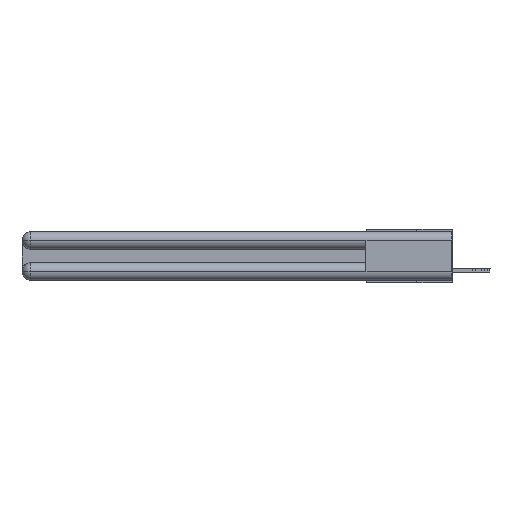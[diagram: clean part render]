
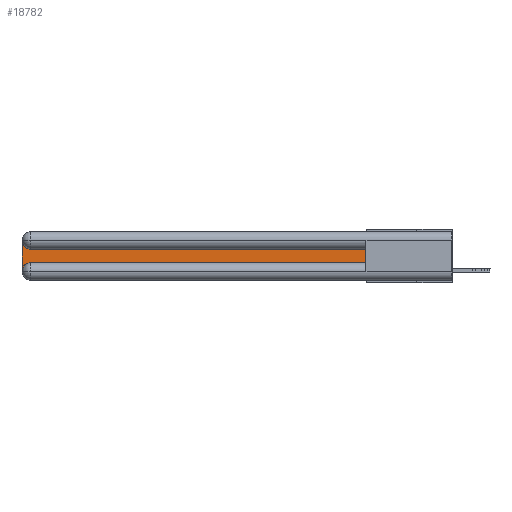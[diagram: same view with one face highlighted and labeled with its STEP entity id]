
A CAD part, left-side view. The second image highlights one B-rep face of the part: STEP entity #18782.
In plain terms, the highlighted planar face has unit normal (-1, 0, 0).
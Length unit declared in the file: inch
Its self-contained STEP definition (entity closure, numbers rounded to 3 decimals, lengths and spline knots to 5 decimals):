
#1051 = PLANE ( 'NONE',  #27890 ) ;
#1833 = LINE ( 'NONE', #15189, #22182 ) ;
#2341 = CARTESIAN_POINT ( 'NONE',  ( 0.075, 3., -0.0625 ) ) ;
#3555 = VERTEX_POINT ( 'NONE', #6981 ) ;
#3709 = EDGE_CURVE ( 'NONE', #29417, #17044, #6085, .T. ) ;
#5444 = DIRECTION ( 'NONE',  ( 0., 0., -1. ) ) ;
#6085 = LINE ( 'NONE', #16145, #34340 ) ;
#6860 = CARTESIAN_POINT ( 'NONE',  ( 0.075, 2.94, -0.2175 ) ) ;
#6981 = CARTESIAN_POINT ( 'NONE',  ( 0.075, 0.6, -0.2175 ) ) ;
#8585 = DIRECTION ( 'NONE',  ( 0., 0., 1. ) ) ;
#9124 = CARTESIAN_POINT ( 'NONE',  ( 0.075, 3., -0.1225 ) ) ;
#10983 = ORIENTED_EDGE ( 'NONE', *, *, #3709, .T. ) ;
#11185 = AXIS2_PLACEMENT_3D ( 'NONE', #26134, #31076, #17866 ) ;
#11230 = FACE_OUTER_BOUND ( 'NONE', #26586, .T. ) ;
#11794 = DIRECTION ( 'NONE',  ( 1., 0., 0. ) ) ;
#11888 = CARTESIAN_POINT ( 'NONE',  ( 0.075, 2.94, -0.0625 ) ) ;
#12434 = VERTEX_POINT ( 'NONE', #13911 ) ;
#13419 = ORIENTED_EDGE ( 'NONE', *, *, #33097, .T. ) ;
#13911 = CARTESIAN_POINT ( 'NONE',  ( 0.075, 2.94, -0.1225 ) ) ;
#14437 = CIRCLE ( 'NONE', #20966, 0.06 ) ;
#15189 = CARTESIAN_POINT ( 'NONE',  ( 0.075, 0.6, -0.2175 ) ) ;
#15497 = CIRCLE ( 'NONE', #11185, 0.06 ) ;
#16033 = VERTEX_POINT ( 'NONE', #26517 ) ;
#16145 = CARTESIAN_POINT ( 'NONE',  ( 0.075, 3., -0.2175 ) ) ;
#17044 = VERTEX_POINT ( 'NONE', #33997 ) ;
#17487 = CARTESIAN_POINT ( 'NONE',  ( 0.075, 0.6, -0.1225 ) ) ;
#17815 = EDGE_CURVE ( 'NONE', #12434, #29417, #14437, .T. ) ;
#17866 = DIRECTION ( 'NONE',  ( 0., 0., -1. ) ) ;
#18782 = ADVANCED_FACE ( 'NONE', ( #11230 ), #1051, .F. ) ;
#19081 = ORIENTED_EDGE ( 'NONE', *, *, #21539, .T. ) ;
#19096 = VECTOR ( 'NONE', #8585, 39.37008 ) ;
#19227 = ORIENTED_EDGE ( 'NONE', *, *, #17815, .T. ) ;
#20371 = DIRECTION ( 'NONE',  ( 0., 1., 0. ) ) ;
#20966 = AXIS2_PLACEMENT_3D ( 'NONE', #11888, #22179, #32943 ) ;
#21373 = VECTOR ( 'NONE', #20371, 39.37008 ) ;
#21539 = EDGE_CURVE ( 'NONE', #16033, #12434, #28452, .T. ) ;
#22179 = DIRECTION ( 'NONE',  ( 1., 0., 0. ) ) ;
#22182 = VECTOR ( 'NONE', #28629, 39.37008 ) ;
#23563 = ORIENTED_EDGE ( 'NONE', *, *, #34323, .T. ) ;
#26134 = CARTESIAN_POINT ( 'NONE',  ( 0.075, 2.94, -0.2775 ) ) ;
#26517 = CARTESIAN_POINT ( 'NONE',  ( 0.075, 0.6, -0.1225 ) ) ;
#26529 = VERTEX_POINT ( 'NONE', #6860 ) ;
#26586 = EDGE_LOOP ( 'NONE', ( #19081, #19227, #10983, #13419, #29066, #23563 ) ) ;
#27027 = LINE ( 'NONE', #27393, #19096 ) ;
#27393 = CARTESIAN_POINT ( 'NONE',  ( 0.075, 0.6, -0.2175 ) ) ;
#27700 = DIRECTION ( 'NONE',  ( 0., 0., -1. ) ) ;
#27890 = AXIS2_PLACEMENT_3D ( 'NONE', #9124, #11794, #27700 ) ;
#28452 = LINE ( 'NONE', #17487, #21373 ) ;
#28629 = DIRECTION ( 'NONE',  ( 0., -1., 0. ) ) ;
#29066 = ORIENTED_EDGE ( 'NONE', *, *, #31209, .T. ) ;
#29417 = VERTEX_POINT ( 'NONE', #2341 ) ;
#31076 = DIRECTION ( 'NONE',  ( 1., 0., 0. ) ) ;
#31209 = EDGE_CURVE ( 'NONE', #26529, #3555, #1833, .T. ) ;
#32943 = DIRECTION ( 'NONE',  ( 0., 0., -1. ) ) ;
#33097 = EDGE_CURVE ( 'NONE', #17044, #26529, #15497, .T. ) ;
#33997 = CARTESIAN_POINT ( 'NONE',  ( 0.075, 3., -0.2775 ) ) ;
#34323 = EDGE_CURVE ( 'NONE', #3555, #16033, #27027, .T. ) ;
#34340 = VECTOR ( 'NONE', #5444, 39.37008 ) ;
